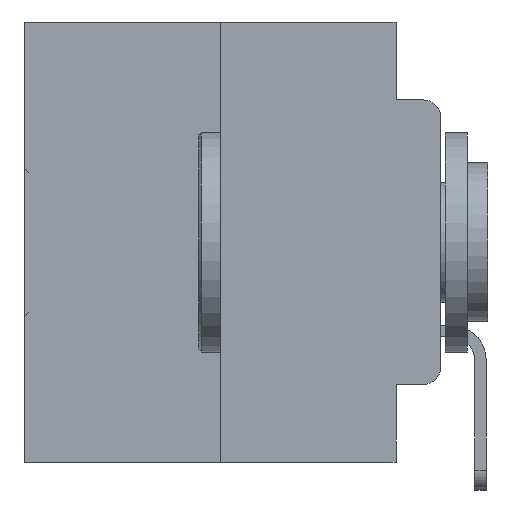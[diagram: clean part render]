
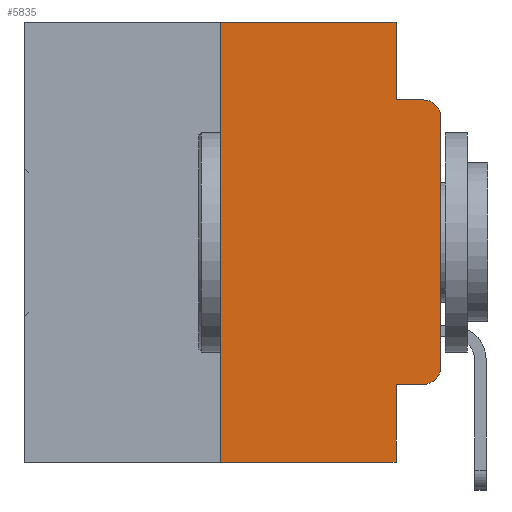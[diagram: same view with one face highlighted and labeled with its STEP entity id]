
A CAD part, left-side view. The second image highlights one B-rep face of the part: STEP entity #5835.
In plain terms, the highlighted planar face has unit normal (-1, 0, 0).
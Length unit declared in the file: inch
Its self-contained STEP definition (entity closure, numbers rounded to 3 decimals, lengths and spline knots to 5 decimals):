
#271 = FACE_OUTER_BOUND ( 'NONE', #3781, .T. ) ;
#667 = CARTESIAN_POINT ( 'NONE',  ( 0., 0.25, 0. ) ) ;
#1015 = VERTEX_POINT ( 'NONE', #16769 ) ;
#1764 = EDGE_CURVE ( 'NONE', #25265, #14924, #24410, .T. ) ;
#2027 = EDGE_CURVE ( 'NONE', #28084, #12714, #21791, .T. ) ;
#2220 = ORIENTED_EDGE ( 'NONE', *, *, #15660, .F. ) ;
#2696 = CARTESIAN_POINT ( 'NONE',  ( 0., 0., -0.1085 ) ) ;
#2859 = AXIS2_PLACEMENT_3D ( 'NONE', #20013, #5130, #22395 ) ;
#3781 = EDGE_LOOP ( 'NONE', ( #26061, #11496, #2220, #15383, #4277, #20242, #29465, #23987, #15853, #10103 ) ) ;
#3977 = VERTEX_POINT ( 'NONE', #4247 ) ;
#4242 = CARTESIAN_POINT ( 'NONE',  ( 0., 0.473, -0.5 ) ) ;
#4247 = CARTESIAN_POINT ( 'NONE',  ( 0., 0.25, 0. ) ) ;
#4277 = ORIENTED_EDGE ( 'NONE', *, *, #7338, .F. ) ;
#5130 = DIRECTION ( 'NONE',  ( -1., 0., 0. ) ) ;
#5748 = VECTOR ( 'NONE', #16650, 39.37008 ) ;
#5835 = ADVANCED_FACE ( 'NONE', ( #271 ), #18196, .F. ) ;
#6714 = DIRECTION ( 'NONE',  ( 0., -1., 0. ) ) ;
#6986 = DIRECTION ( 'NONE',  ( 0., 0., -1. ) ) ;
#7338 = EDGE_CURVE ( 'NONE', #3977, #28084, #12439, .T. ) ;
#7829 = CIRCLE ( 'NONE', #10982, 0.02 ) ;
#8442 = CARTESIAN_POINT ( 'NONE',  ( 0., 0.051, -0.4115 ) ) ;
#8603 = AXIS2_PLACEMENT_3D ( 'NONE', #15797, #25245, #20573 ) ;
#10103 = ORIENTED_EDGE ( 'NONE', *, *, #30680, .T. ) ;
#10296 = EDGE_CURVE ( 'NONE', #11416, #14924, #20807, .T. ) ;
#10650 = CARTESIAN_POINT ( 'NONE',  ( 0., 0., -0.3915 ) ) ;
#10708 = CARTESIAN_POINT ( 'NONE',  ( 0., 0.02, -0.1085 ) ) ;
#10714 = CARTESIAN_POINT ( 'NONE',  ( 0., 0., 0. ) ) ;
#10975 = CARTESIAN_POINT ( 'NONE',  ( 0., 0.051, 0. ) ) ;
#10982 = AXIS2_PLACEMENT_3D ( 'NONE', #10708, #27494, #13273 ) ;
#11416 = VERTEX_POINT ( 'NONE', #19592 ) ;
#11496 = ORIENTED_EDGE ( 'NONE', *, *, #14899, .T. ) ;
#12439 = LINE ( 'NONE', #22344, #24385 ) ;
#12714 = VERTEX_POINT ( 'NONE', #19951 ) ;
#13273 = DIRECTION ( 'NONE',  ( 0., 0., -1. ) ) ;
#13683 = LINE ( 'NONE', #667, #31122 ) ;
#13849 = CARTESIAN_POINT ( 'NONE',  ( 0., 0.051, 0. ) ) ;
#14729 = VECTOR ( 'NONE', #6986, 39.37008 ) ;
#14899 = EDGE_CURVE ( 'NONE', #23017, #1015, #7829, .T. ) ;
#14924 = VERTEX_POINT ( 'NONE', #29878 ) ;
#15022 = VECTOR ( 'NONE', #29887, 39.37008 ) ;
#15213 = VERTEX_POINT ( 'NONE', #21964 ) ;
#15383 = ORIENTED_EDGE ( 'NONE', *, *, #2027, .F. ) ;
#15660 = EDGE_CURVE ( 'NONE', #12714, #1015, #20383, .T. ) ;
#15797 = CARTESIAN_POINT ( 'NONE',  ( 0., 0.473, 0. ) ) ;
#15853 = ORIENTED_EDGE ( 'NONE', *, *, #31093, .T. ) ;
#16003 = CIRCLE ( 'NONE', #2859, 0.02 ) ;
#16650 = DIRECTION ( 'NONE',  ( 0., -1., 0. ) ) ;
#16769 = CARTESIAN_POINT ( 'NONE',  ( 0., 0.02, -0.0885 ) ) ;
#17856 = VERTEX_POINT ( 'NONE', #10650 ) ;
#18196 = PLANE ( 'NONE',  #8603 ) ;
#18303 = DIRECTION ( 'NONE',  ( 0., 0., -1. ) ) ;
#19592 = CARTESIAN_POINT ( 'NONE',  ( 0., 0.25, -0.5 ) ) ;
#19951 = CARTESIAN_POINT ( 'NONE',  ( 0., 0.051, -0.0885 ) ) ;
#20013 = CARTESIAN_POINT ( 'NONE',  ( 0., 0.02, -0.3915 ) ) ;
#20074 = VECTOR ( 'NONE', #6714, 39.37008 ) ;
#20242 = ORIENTED_EDGE ( 'NONE', *, *, #27393, .F. ) ;
#20383 = LINE ( 'NONE', #21201, #25937 ) ;
#20573 = DIRECTION ( 'NONE',  ( 0., 0., -1. ) ) ;
#20807 = LINE ( 'NONE', #4242, #20074 ) ;
#21201 = CARTESIAN_POINT ( 'NONE',  ( 0., 0.051, -0.0885 ) ) ;
#21791 = LINE ( 'NONE', #31126, #14729 ) ;
#21964 = CARTESIAN_POINT ( 'NONE',  ( 0., 0.02, -0.4115 ) ) ;
#22090 = LINE ( 'NONE', #10714, #15022 ) ;
#22344 = CARTESIAN_POINT ( 'NONE',  ( 0., 0.473, 0. ) ) ;
#22395 = DIRECTION ( 'NONE',  ( 0., 0., -1. ) ) ;
#23017 = VERTEX_POINT ( 'NONE', #2696 ) ;
#23047 = DIRECTION ( 'NONE',  ( 0., 0., 1. ) ) ;
#23099 = EDGE_CURVE ( 'NONE', #17856, #23017, #22090, .T. ) ;
#23595 = DIRECTION ( 'NONE',  ( 0., -1., 0. ) ) ;
#23673 = VECTOR ( 'NONE', #18303, 39.37008 ) ;
#23987 = ORIENTED_EDGE ( 'NONE', *, *, #1764, .F. ) ;
#24385 = VECTOR ( 'NONE', #27098, 39.37008 ) ;
#24410 = LINE ( 'NONE', #10975, #23673 ) ;
#24524 = LINE ( 'NONE', #30849, #5748 ) ;
#25245 = DIRECTION ( 'NONE',  ( 1., 0., 0. ) ) ;
#25265 = VERTEX_POINT ( 'NONE', #8442 ) ;
#25937 = VECTOR ( 'NONE', #23595, 39.37008 ) ;
#26061 = ORIENTED_EDGE ( 'NONE', *, *, #23099, .T. ) ;
#27098 = DIRECTION ( 'NONE',  ( 0., -1., 0. ) ) ;
#27393 = EDGE_CURVE ( 'NONE', #11416, #3977, #13683, .T. ) ;
#27494 = DIRECTION ( 'NONE',  ( -1., 0., 0. ) ) ;
#28084 = VERTEX_POINT ( 'NONE', #13849 ) ;
#29465 = ORIENTED_EDGE ( 'NONE', *, *, #10296, .T. ) ;
#29878 = CARTESIAN_POINT ( 'NONE',  ( 0., 0.051, -0.5 ) ) ;
#29887 = DIRECTION ( 'NONE',  ( 0., 0., 1. ) ) ;
#30680 = EDGE_CURVE ( 'NONE', #15213, #17856, #16003, .T. ) ;
#30849 = CARTESIAN_POINT ( 'NONE',  ( 0., 0.051, -0.4115 ) ) ;
#31093 = EDGE_CURVE ( 'NONE', #25265, #15213, #24524, .T. ) ;
#31122 = VECTOR ( 'NONE', #23047, 39.37008 ) ;
#31126 = CARTESIAN_POINT ( 'NONE',  ( 0., 0.051, 0. ) ) ;
